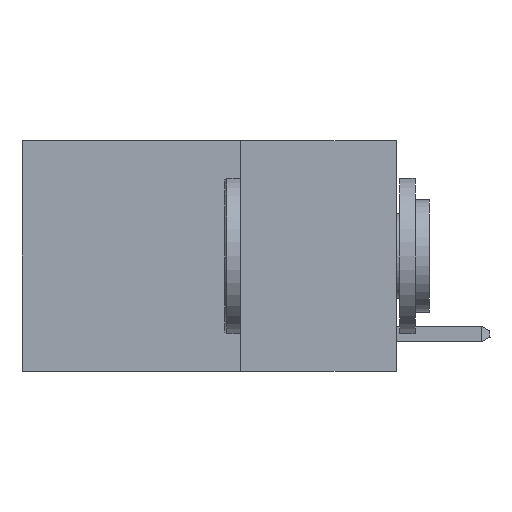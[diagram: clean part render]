
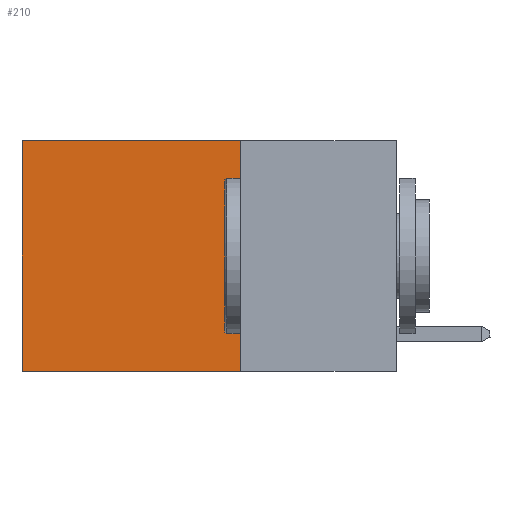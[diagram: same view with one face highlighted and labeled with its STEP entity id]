
A CAD part, left-side view. The second image highlights one B-rep face of the part: STEP entity #210.
In plain terms, the highlighted planar face has unit normal (-1, 0, 0).
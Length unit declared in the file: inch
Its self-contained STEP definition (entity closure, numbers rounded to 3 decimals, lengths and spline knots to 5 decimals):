
#210 = ADVANCED_FACE ( 'NONE', ( #5428 ), #13837, .F. ) ;
#849 = ORIENTED_EDGE ( 'NONE', *, *, #1038, .F. ) ;
#1038 = EDGE_CURVE ( 'NONE', #22512, #6816, #3638, .T. ) ;
#3195 = EDGE_CURVE ( 'NONE', #6816, #12711, #23938, .T. ) ;
#3466 = AXIS2_PLACEMENT_3D ( 'NONE', #22208, #4069, #14379 ) ;
#3575 = CARTESIAN_POINT ( 'NONE',  ( 0.2625, 0.6, 0. ) ) ;
#3638 = LINE ( 'NONE', #17931, #24578 ) ;
#4069 = DIRECTION ( 'NONE',  ( 1., 0., 0. ) ) ;
#5428 = FACE_OUTER_BOUND ( 'NONE', #19085, .T. ) ;
#6036 = CARTESIAN_POINT ( 'NONE',  ( 0.2625, 0.25, -0.37 ) ) ;
#6816 = VERTEX_POINT ( 'NONE', #6036 ) ;
#8262 = LINE ( 'NONE', #26982, #26892 ) ;
#8546 = VECTOR ( 'NONE', #13122, 39.37008 ) ;
#8700 = CARTESIAN_POINT ( 'NONE',  ( 0.2625, 0.6, 0. ) ) ;
#9230 = CARTESIAN_POINT ( 'NONE',  ( 0.2625, 0.25, 0. ) ) ;
#9482 = DIRECTION ( 'NONE',  ( 0., 1., 0. ) ) ;
#12711 = VERTEX_POINT ( 'NONE', #19106 ) ;
#12821 = ORIENTED_EDGE ( 'NONE', *, *, #3195, .F. ) ;
#13122 = DIRECTION ( 'NONE',  ( 0., 0., -1. ) ) ;
#13618 = CARTESIAN_POINT ( 'NONE',  ( 0.2625, 0.25, -0.37 ) ) ;
#13837 = PLANE ( 'NONE',  #3466 ) ;
#14379 = DIRECTION ( 'NONE',  ( 0., 0., -1. ) ) ;
#15024 = ORIENTED_EDGE ( 'NONE', *, *, #19162, .T. ) ;
#16671 = DIRECTION ( 'NONE',  ( 0., 1., 0. ) ) ;
#17931 = CARTESIAN_POINT ( 'NONE',  ( 0.2625, 0.25, 0. ) ) ;
#19085 = EDGE_LOOP ( 'NONE', ( #27034, #12821, #849, #15024 ) ) ;
#19106 = CARTESIAN_POINT ( 'NONE',  ( 0.2625, 0.6, -0.37 ) ) ;
#19162 = EDGE_CURVE ( 'NONE', #22512, #26529, #8262, .T. ) ;
#19718 = DIRECTION ( 'NONE',  ( 0., 0., -1. ) ) ;
#21222 = LINE ( 'NONE', #8700, #8546 ) ;
#21618 = VECTOR ( 'NONE', #9482, 39.37008 ) ;
#22067 = EDGE_CURVE ( 'NONE', #26529, #12711, #21222, .T. ) ;
#22208 = CARTESIAN_POINT ( 'NONE',  ( 0.2625, 0.25, 0. ) ) ;
#22512 = VERTEX_POINT ( 'NONE', #9230 ) ;
#23938 = LINE ( 'NONE', #13618, #21618 ) ;
#24578 = VECTOR ( 'NONE', #19718, 39.37008 ) ;
#26529 = VERTEX_POINT ( 'NONE', #3575 ) ;
#26892 = VECTOR ( 'NONE', #16671, 39.37008 ) ;
#26982 = CARTESIAN_POINT ( 'NONE',  ( 0.2625, 0.25, 0. ) ) ;
#27034 = ORIENTED_EDGE ( 'NONE', *, *, #22067, .T. ) ;
